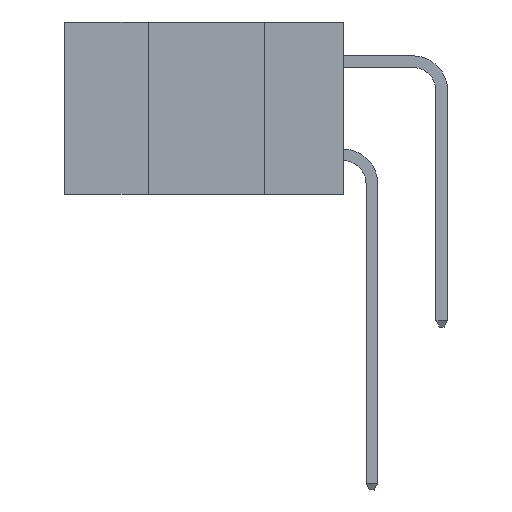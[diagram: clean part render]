
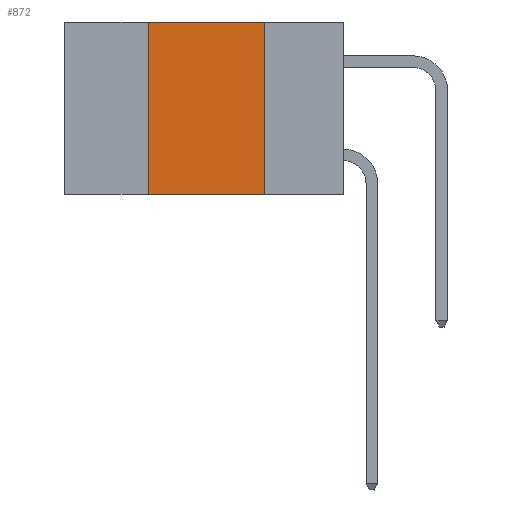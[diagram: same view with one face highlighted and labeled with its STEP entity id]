
A CAD part, left-side view. The second image highlights one B-rep face of the part: STEP entity #872.
In plain terms, the highlighted planar face has unit normal (-1, 0, 0).
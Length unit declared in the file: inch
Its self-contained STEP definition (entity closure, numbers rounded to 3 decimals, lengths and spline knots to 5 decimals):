
#200 = ORIENTED_EDGE ( 'NONE', *, *, #3137, .F. ) ;
#666 = CARTESIAN_POINT ( 'NONE',  ( 0., 0.17, 0. ) ) ;
#872 = ADVANCED_FACE ( 'NONE', ( #13364 ), #4569, .F. ) ;
#1073 = CARTESIAN_POINT ( 'NONE',  ( 0., 0.17, 0. ) ) ;
#1888 = ORIENTED_EDGE ( 'NONE', *, *, #7028, .T. ) ;
#2405 = DIRECTION ( 'NONE',  ( 1., 0., 0. ) ) ;
#2566 = DIRECTION ( 'NONE',  ( 0., -1., 0. ) ) ;
#2849 = CARTESIAN_POINT ( 'NONE',  ( 0., 0.6, -0.37 ) ) ;
#3137 = EDGE_CURVE ( 'NONE', #6406, #3643, #11208, .T. ) ;
#3643 = VERTEX_POINT ( 'NONE', #5499 ) ;
#4569 = PLANE ( 'NONE',  #12276 ) ;
#5063 = EDGE_LOOP ( 'NONE', ( #200, #9569, #9751, #1888 ) ) ;
#5247 = VECTOR ( 'NONE', #2566, 39.37008 ) ;
#5499 = CARTESIAN_POINT ( 'NONE',  ( 0., 0.17, -0.37 ) ) ;
#5738 = LINE ( 'NONE', #8523, #12360 ) ;
#6073 = VERTEX_POINT ( 'NONE', #11704 ) ;
#6406 = VERTEX_POINT ( 'NONE', #666 ) ;
#6510 = DIRECTION ( 'NONE',  ( 0., 0., 1. ) ) ;
#7028 = EDGE_CURVE ( 'NONE', #6073, #3643, #8395, .T. ) ;
#7155 = DIRECTION ( 'NONE',  ( 0., -1., 0. ) ) ;
#7635 = EDGE_CURVE ( 'NONE', #6073, #11011, #5738, .T. ) ;
#7705 = CARTESIAN_POINT ( 'NONE',  ( 0., 0.42, 0. ) ) ;
#7939 = CARTESIAN_POINT ( 'NONE',  ( 0., 0.6, 0. ) ) ;
#8395 = LINE ( 'NONE', #2849, #11046 ) ;
#8472 = DIRECTION ( 'NONE',  ( 0., 0., -1. ) ) ;
#8523 = CARTESIAN_POINT ( 'NONE',  ( 0., 0.42, 0. ) ) ;
#9363 = LINE ( 'NONE', #11937, #5247 ) ;
#9569 = ORIENTED_EDGE ( 'NONE', *, *, #10449, .F. ) ;
#9751 = ORIENTED_EDGE ( 'NONE', *, *, #7635, .F. ) ;
#10449 = EDGE_CURVE ( 'NONE', #11011, #6406, #9363, .T. ) ;
#11011 = VERTEX_POINT ( 'NONE', #7705 ) ;
#11046 = VECTOR ( 'NONE', #7155, 39.37008 ) ;
#11208 = LINE ( 'NONE', #1073, #13375 ) ;
#11704 = CARTESIAN_POINT ( 'NONE',  ( 0., 0.42, -0.37 ) ) ;
#11937 = CARTESIAN_POINT ( 'NONE',  ( 0., 0.6, 0. ) ) ;
#11973 = DIRECTION ( 'NONE',  ( 0., 0., -1. ) ) ;
#12276 = AXIS2_PLACEMENT_3D ( 'NONE', #7939, #2405, #11973 ) ;
#12360 = VECTOR ( 'NONE', #6510, 39.37008 ) ;
#13364 = FACE_OUTER_BOUND ( 'NONE', #5063, .T. ) ;
#13375 = VECTOR ( 'NONE', #8472, 39.37008 ) ;
